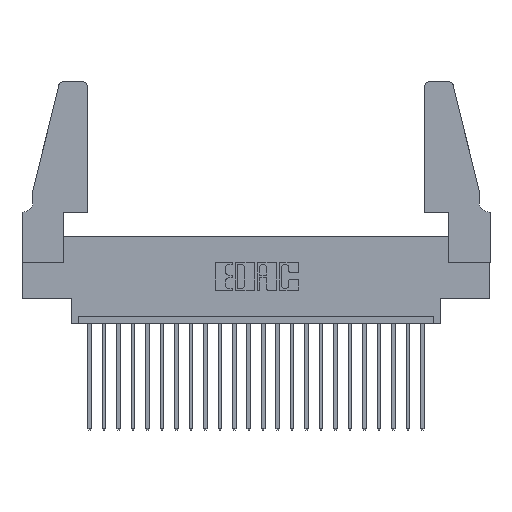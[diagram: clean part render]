
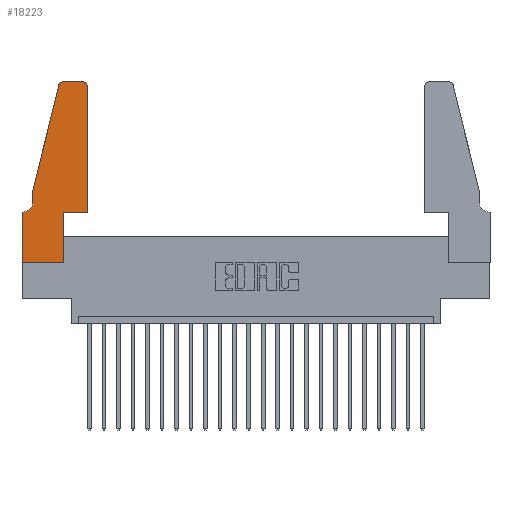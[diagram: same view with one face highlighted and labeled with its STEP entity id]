
A CAD part, top view. The second image highlights one B-rep face of the part: STEP entity #18223.
In plain terms, the highlighted planar face has unit normal (0, 0, 1).
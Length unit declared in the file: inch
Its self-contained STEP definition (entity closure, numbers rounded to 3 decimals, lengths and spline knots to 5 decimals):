
#15 = FACE_OUTER_BOUND ( 'NONE', #11046, .T. ) ;
#57 = CIRCLE ( 'NONE', #19970, 0.03 ) ;
#375 = ORIENTED_EDGE ( 'NONE', *, *, #11625, .T. ) ;
#383 = CARTESIAN_POINT ( 'NONE',  ( 0.4505, 0.35, 0.37 ) ) ;
#385 = DIRECTION ( 'NONE',  ( -0.239, -0.971, 0. ) ) ;
#423 = CARTESIAN_POINT ( 'NONE',  ( 0.0055, 0.42, 0.37 ) ) ;
#887 = DIRECTION ( 'NONE',  ( 1., 0., 0. ) ) ;
#970 = ORIENTED_EDGE ( 'NONE', *, *, #5577, .T. ) ;
#996 = EDGE_CURVE ( 'NONE', #14188, #1510, #22374, .T. ) ;
#1053 = VERTEX_POINT ( 'NONE', #16963 ) ;
#1510 = VERTEX_POINT ( 'NONE', #9375 ) ;
#1578 = CARTESIAN_POINT ( 'NONE',  ( 0.2865, 0., 0.37 ) ) ;
#2097 = CIRCLE ( 'NONE', #11373, 0.07 ) ;
#2240 = DIRECTION ( 'NONE',  ( 1., 0., 0. ) ) ;
#2243 = VERTEX_POINT ( 'NONE', #9502 ) ;
#2959 = VECTOR ( 'NONE', #10990, 39.37008 ) ;
#3500 = LINE ( 'NONE', #16882, #7072 ) ;
#3664 = CARTESIAN_POINT ( 'NONE',  ( 0.4505, 1.22, 0.37 ) ) ;
#3785 = EDGE_CURVE ( 'NONE', #1053, #2243, #11041, .T. ) ;
#4004 = CARTESIAN_POINT ( 'NONE',  ( 0.0055, 0.35, 0.37 ) ) ;
#4245 = VERTEX_POINT ( 'NONE', #16250 ) ;
#4398 = DIRECTION ( 'NONE',  ( 0., -1., 0. ) ) ;
#4570 = VERTEX_POINT ( 'NONE', #3664 ) ;
#4681 = VECTOR ( 'NONE', #18029, 39.37008 ) ;
#5158 = EDGE_CURVE ( 'NONE', #11365, #4570, #16714, .T. ) ;
#5524 = CARTESIAN_POINT ( 'NONE',  ( 0., 0., 0.37 ) ) ;
#5577 = EDGE_CURVE ( 'NONE', #12670, #11365, #19667, .T. ) ;
#5691 = PLANE ( 'NONE',  #8385 ) ;
#6096 = ORIENTED_EDGE ( 'NONE', *, *, #16883, .T. ) ;
#6103 = CARTESIAN_POINT ( 'NONE',  ( 0., 0., 0.37 ) ) ;
#6183 = ORIENTED_EDGE ( 'NONE', *, *, #18179, .T. ) ;
#6766 = VECTOR ( 'NONE', #2240, 39.37008 ) ;
#6825 = CARTESIAN_POINT ( 'NONE',  ( 0.0755, 0.35, 0.37 ) ) ;
#6858 = VECTOR ( 'NONE', #385, 39.37008 ) ;
#6891 = VERTEX_POINT ( 'NONE', #20845 ) ;
#7072 = VECTOR ( 'NONE', #13331, 39.37008 ) ;
#7257 = CARTESIAN_POINT ( 'NONE',  ( 0.2865, 0.35, 0.37 ) ) ;
#7415 = CARTESIAN_POINT ( 'NONE',  ( 0.2865, 0.35, 0.37 ) ) ;
#7420 = CARTESIAN_POINT ( 'NONE',  ( 0.2605, 1.25, 0.37 ) ) ;
#7615 = CARTESIAN_POINT ( 'NONE',  ( 0.284, 1.22, 0.37 ) ) ;
#7755 = ORIENTED_EDGE ( 'NONE', *, *, #9632, .T. ) ;
#8135 = VERTEX_POINT ( 'NONE', #8629 ) ;
#8385 = AXIS2_PLACEMENT_3D ( 'NONE', #12533, #19479, #9071 ) ;
#8587 = LINE ( 'NONE', #6103, #17363 ) ;
#8629 = CARTESIAN_POINT ( 'NONE',  ( 0., 0., 0.37 ) ) ;
#9071 = DIRECTION ( 'NONE',  ( 1., 0., 0. ) ) ;
#9152 = DIRECTION ( 'NONE',  ( -1., 0., 0. ) ) ;
#9244 = EDGE_CURVE ( 'NONE', #4570, #1053, #18561, .T. ) ;
#9304 = AXIS2_PLACEMENT_3D ( 'NONE', #9629, #16430, #887 ) ;
#9375 = CARTESIAN_POINT ( 'NONE',  ( 0., 0.35, 0.37 ) ) ;
#9491 = VECTOR ( 'NONE', #10916, 39.37008 ) ;
#9502 = CARTESIAN_POINT ( 'NONE',  ( 0.284, 1.25, 0.37 ) ) ;
#9590 = ORIENTED_EDGE ( 'NONE', *, *, #19283, .T. ) ;
#9603 = ORIENTED_EDGE ( 'NONE', *, *, #14733, .T. ) ;
#9629 = CARTESIAN_POINT ( 'NONE',  ( 0.4205, 1.22, 0.37 ) ) ;
#9632 = EDGE_CURVE ( 'NONE', #8135, #11512, #18786, .T. ) ;
#9888 = LINE ( 'NONE', #7415, #2959 ) ;
#10916 = DIRECTION ( 'NONE',  ( 1., 0., 0. ) ) ;
#10990 = DIRECTION ( 'NONE',  ( 0., 1., 0. ) ) ;
#11041 = LINE ( 'NONE', #7420, #4681 ) ;
#11046 = EDGE_LOOP ( 'NONE', ( #11444, #6096, #375, #9590, #22780, #17691, #6183, #7755, #9603, #970, #16691, #15836 ) ) ;
#11365 = VERTEX_POINT ( 'NONE', #383 ) ;
#11373 = AXIS2_PLACEMENT_3D ( 'NONE', #423, #19730, #12699 ) ;
#11444 = ORIENTED_EDGE ( 'NONE', *, *, #3785, .T. ) ;
#11512 = VERTEX_POINT ( 'NONE', #1578 ) ;
#11625 = EDGE_CURVE ( 'NONE', #4245, #6891, #20584, .T. ) ;
#12041 = VECTOR ( 'NONE', #22475, 39.37008 ) ;
#12533 = CARTESIAN_POINT ( 'NONE',  ( 0., 0.35, 0.37 ) ) ;
#12670 = VERTEX_POINT ( 'NONE', #7257 ) ;
#12699 = DIRECTION ( 'NONE',  ( -1., 0., 0. ) ) ;
#13331 = DIRECTION ( 'NONE',  ( 0., -1., 0. ) ) ;
#14188 = VERTEX_POINT ( 'NONE', #4004 ) ;
#14513 = CARTESIAN_POINT ( 'NONE',  ( 0.0755, 0.5, 0.37 ) ) ;
#14733 = EDGE_CURVE ( 'NONE', #11512, #12670, #9888, .T. ) ;
#15010 = VERTEX_POINT ( 'NONE', #21569 ) ;
#15836 = ORIENTED_EDGE ( 'NONE', *, *, #9244, .T. ) ;
#16250 = CARTESIAN_POINT ( 'NONE',  ( 0.25487, 1.22718, 0.37 ) ) ;
#16430 = DIRECTION ( 'NONE',  ( 0., 0., 1. ) ) ;
#16601 = DIRECTION ( 'NONE',  ( 0., 0., 1. ) ) ;
#16665 = CARTESIAN_POINT ( 'NONE',  ( 0.4505, 0.35, 0.37 ) ) ;
#16691 = ORIENTED_EDGE ( 'NONE', *, *, #5158, .T. ) ;
#16714 = LINE ( 'NONE', #16665, #12041 ) ;
#16882 = CARTESIAN_POINT ( 'NONE',  ( 0.0755, 0.5, 0.37 ) ) ;
#16883 = EDGE_CURVE ( 'NONE', #2243, #4245, #57, .T. ) ;
#16963 = CARTESIAN_POINT ( 'NONE',  ( 0.4205, 1.25, 0.37 ) ) ;
#17363 = VECTOR ( 'NONE', #4398, 39.37008 ) ;
#17691 = ORIENTED_EDGE ( 'NONE', *, *, #996, .T. ) ;
#17987 = CARTESIAN_POINT ( 'NONE',  ( 0.4505, 0.35, 0.37 ) ) ;
#18029 = DIRECTION ( 'NONE',  ( -1., 0., 0. ) ) ;
#18179 = EDGE_CURVE ( 'NONE', #1510, #8135, #8587, .T. ) ;
#18223 = ADVANCED_FACE ( 'NONE', ( #15 ), #5691, .T. ) ;
#18561 = CIRCLE ( 'NONE', #9304, 0.03 ) ;
#18786 = LINE ( 'NONE', #5524, #9491 ) ;
#19283 = EDGE_CURVE ( 'NONE', #6891, #15010, #3500, .T. ) ;
#19479 = DIRECTION ( 'NONE',  ( 0., 0., 1. ) ) ;
#19667 = LINE ( 'NONE', #17987, #6766 ) ;
#19730 = DIRECTION ( 'NONE',  ( 0., 0., -1. ) ) ;
#19970 = AXIS2_PLACEMENT_3D ( 'NONE', #7615, #16601, #21745 ) ;
#19974 = EDGE_CURVE ( 'NONE', #15010, #14188, #2097, .T. ) ;
#20584 = LINE ( 'NONE', #14513, #6858 ) ;
#20845 = CARTESIAN_POINT ( 'NONE',  ( 0.0755, 0.5, 0.37 ) ) ;
#21569 = CARTESIAN_POINT ( 'NONE',  ( 0.0755, 0.42, 0.37 ) ) ;
#21745 = DIRECTION ( 'NONE',  ( 1., 0., 0. ) ) ;
#22102 = VECTOR ( 'NONE', #9152, 39.37008 ) ;
#22374 = LINE ( 'NONE', #6825, #22102 ) ;
#22475 = DIRECTION ( 'NONE',  ( 0., 1., 0. ) ) ;
#22780 = ORIENTED_EDGE ( 'NONE', *, *, #19974, .T. ) ;
